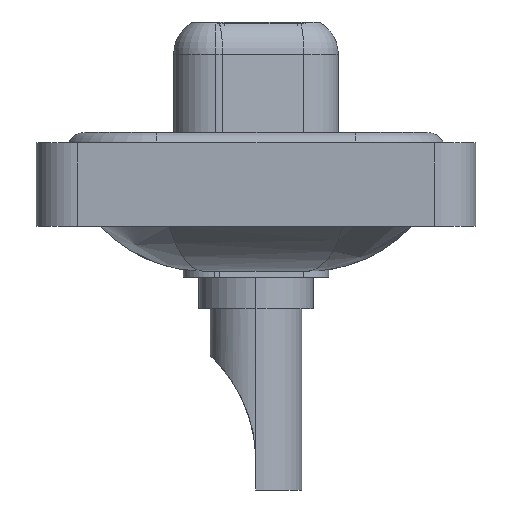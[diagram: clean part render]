
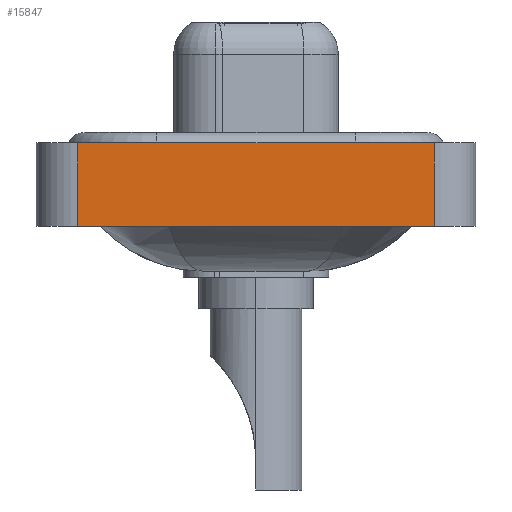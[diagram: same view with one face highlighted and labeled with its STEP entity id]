
A CAD part, left-side view. The second image highlights one B-rep face of the part: STEP entity #15847.
In plain terms, the highlighted planar face has unit normal (-1, 0, 0).
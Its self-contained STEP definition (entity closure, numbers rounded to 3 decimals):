
#553 = EDGE_LOOP ( 'NONE', ( #10931, #10552, #15518, #19519 ) ) ;
#967 = VERTEX_POINT ( 'NONE', #20507 ) ;
#1000 = CARTESIAN_POINT ( 'NONE',  ( -7.3, 8.55, -3.6 ) ) ;
#1670 = DIRECTION ( 'NONE',  ( 0., 0., 1. ) ) ;
#3966 = CARTESIAN_POINT ( 'NONE',  ( -7.3, -8.55, -3.6 ) ) ;
#3976 = DIRECTION ( 'NONE',  ( -1., 0., 0. ) ) ;
#4166 = VECTOR ( 'NONE', #12535, 1000. ) ;
#4178 = EDGE_CURVE ( 'NONE', #16613, #19757, #13623, .T. ) ;
#4405 = CARTESIAN_POINT ( 'NONE',  ( -7.3, 8.55, -3.6 ) ) ;
#5564 = PLANE ( 'NONE',  #17310 ) ;
#5690 = EDGE_CURVE ( 'NONE', #16613, #6799, #15648, .T. ) ;
#6179 = CARTESIAN_POINT ( 'NONE',  ( -7.3, -8.55, -3.6 ) ) ;
#6586 = CARTESIAN_POINT ( 'NONE',  ( -7.3, -8.55, -3.6 ) ) ;
#6733 = CARTESIAN_POINT ( 'NONE',  ( -7.3, 8.55, 0.4 ) ) ;
#6799 = VERTEX_POINT ( 'NONE', #3966 ) ;
#7368 = DIRECTION ( 'NONE',  ( 0., 0., 1. ) ) ;
#8129 = LINE ( 'NONE', #6586, #11859 ) ;
#10552 = ORIENTED_EDGE ( 'NONE', *, *, #12645, .F. ) ;
#10931 = ORIENTED_EDGE ( 'NONE', *, *, #20598, .T. ) ;
#11859 = VECTOR ( 'NONE', #17701, 1000. ) ;
#11913 = CARTESIAN_POINT ( 'NONE',  ( -7.3, -8.55, -3.6 ) ) ;
#12535 = DIRECTION ( 'NONE',  ( 0., -1., 0. ) ) ;
#12645 = EDGE_CURVE ( 'NONE', #19757, #967, #14256, .T. ) ;
#12701 = CARTESIAN_POINT ( 'NONE',  ( -7.3, -8.55, 0.4 ) ) ;
#13383 = VECTOR ( 'NONE', #19041, 1000. ) ;
#13623 = LINE ( 'NONE', #1000, #14868 ) ;
#14256 = LINE ( 'NONE', #12701, #13383 ) ;
#14868 = VECTOR ( 'NONE', #7368, 1000. ) ;
#15518 = ORIENTED_EDGE ( 'NONE', *, *, #4178, .F. ) ;
#15648 = LINE ( 'NONE', #6179, #4166 ) ;
#15847 = ADVANCED_FACE ( 'NONE', ( #16979 ), #5564, .T. ) ;
#16613 = VERTEX_POINT ( 'NONE', #4405 ) ;
#16979 = FACE_OUTER_BOUND ( 'NONE', #553, .T. ) ;
#17310 = AXIS2_PLACEMENT_3D ( 'NONE', #11913, #3976, #1670 ) ;
#17701 = DIRECTION ( 'NONE',  ( 0., 0., 1. ) ) ;
#19041 = DIRECTION ( 'NONE',  ( 0., -1., 0. ) ) ;
#19519 = ORIENTED_EDGE ( 'NONE', *, *, #5690, .T. ) ;
#19757 = VERTEX_POINT ( 'NONE', #6733 ) ;
#20507 = CARTESIAN_POINT ( 'NONE',  ( -7.3, -8.55, 0.4 ) ) ;
#20598 = EDGE_CURVE ( 'NONE', #6799, #967, #8129, .T. ) ;
